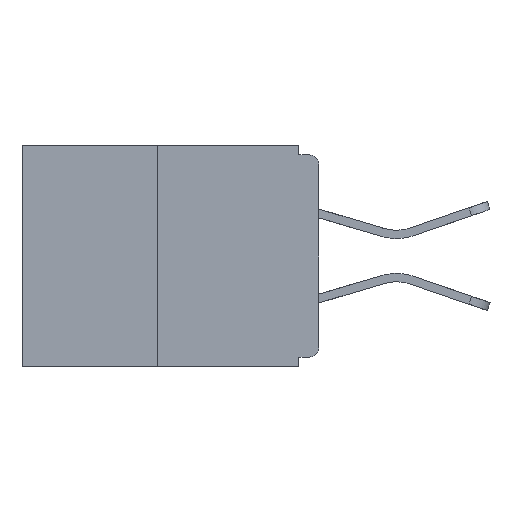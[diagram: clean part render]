
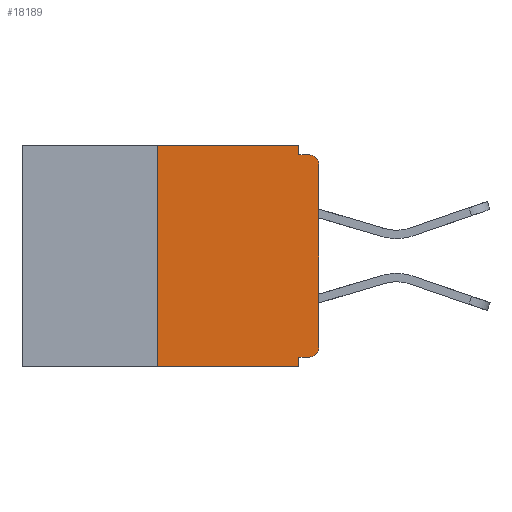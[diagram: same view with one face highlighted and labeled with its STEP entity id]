
A CAD part, left-side view. The second image highlights one B-rep face of the part: STEP entity #18189.
In plain terms, the highlighted planar face has unit normal (-1, 0, 0).
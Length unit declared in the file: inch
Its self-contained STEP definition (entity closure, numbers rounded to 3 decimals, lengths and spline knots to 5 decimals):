
#52 = VERTEX_POINT ( 'NONE', #10032 ) ;
#620 = CARTESIAN_POINT ( 'NONE',  ( 0., 0.015, -0.03 ) ) ;
#627 = DIRECTION ( 'NONE',  ( 0., 1., 0. ) ) ;
#785 = DIRECTION ( 'NONE',  ( 0., -1., 0. ) ) ;
#1181 = VECTOR ( 'NONE', #5397, 39.37008 ) ;
#1182 = AXIS2_PLACEMENT_3D ( 'NONE', #11232, #16362, #14877 ) ;
#1285 = CARTESIAN_POINT ( 'NONE',  ( 0., 0.015, -0.313 ) ) ;
#1603 = VECTOR ( 'NONE', #8721, 39.37008 ) ;
#1796 = EDGE_CURVE ( 'NONE', #11102, #2314, #11793, .T. ) ;
#2314 = VERTEX_POINT ( 'NONE', #2951 ) ;
#2432 = LINE ( 'NONE', #12105, #1603 ) ;
#2464 = PLANE ( 'NONE',  #1182 ) ;
#2807 = CARTESIAN_POINT ( 'NONE',  ( 0., 0.25, 0. ) ) ;
#2951 = CARTESIAN_POINT ( 'NONE',  ( 0., 0.031, -0.343 ) ) ;
#3135 = ORIENTED_EDGE ( 'NONE', *, *, #6657, .T. ) ;
#3842 = DIRECTION ( 'NONE',  ( 0., 0., 1. ) ) ;
#4138 = CARTESIAN_POINT ( 'NONE',  ( 0., 0.031, -0.343 ) ) ;
#4311 = EDGE_LOOP ( 'NONE', ( #10356, #5487, #3135, #16318, #19815, #11335, #14753, #18255, #19590, #19221 ) ) ;
#4668 = EDGE_CURVE ( 'NONE', #52, #5228, #10355, .T. ) ;
#4966 = FACE_OUTER_BOUND ( 'NONE', #4311, .T. ) ;
#5228 = VERTEX_POINT ( 'NONE', #5696 ) ;
#5397 = DIRECTION ( 'NONE',  ( 0., -1., 0. ) ) ;
#5487 = ORIENTED_EDGE ( 'NONE', *, *, #22257, .F. ) ;
#5653 = DIRECTION ( 'NONE',  ( 0., 0., -1. ) ) ;
#5679 = CARTESIAN_POINT ( 'NONE',  ( 0., 0., -0.313 ) ) ;
#5696 = CARTESIAN_POINT ( 'NONE',  ( 0., 0.015, -0.015 ) ) ;
#6507 = AXIS2_PLACEMENT_3D ( 'NONE', #1285, #7897, #7832 ) ;
#6517 = LINE ( 'NONE', #17927, #19963 ) ;
#6657 = EDGE_CURVE ( 'NONE', #22185, #2314, #14113, .T. ) ;
#6811 = LINE ( 'NONE', #17687, #15158 ) ;
#7174 = AXIS2_PLACEMENT_3D ( 'NONE', #620, #7460, #5653 ) ;
#7367 = DIRECTION ( 'NONE',  ( 0., 0., -1. ) ) ;
#7460 = DIRECTION ( 'NONE',  ( -1., 0., 0. ) ) ;
#7615 = VERTEX_POINT ( 'NONE', #15777 ) ;
#7832 = DIRECTION ( 'NONE',  ( 0., 0., -1. ) ) ;
#7897 = DIRECTION ( 'NONE',  ( -1., 0., 0. ) ) ;
#8721 = DIRECTION ( 'NONE',  ( 0., -1., 0. ) ) ;
#8995 = VERTEX_POINT ( 'NONE', #2807 ) ;
#9197 = CARTESIAN_POINT ( 'NONE',  ( 0., 0.25, 0. ) ) ;
#9594 = EDGE_CURVE ( 'NONE', #12391, #11303, #10916, .T. ) ;
#10032 = CARTESIAN_POINT ( 'NONE',  ( 0., 0., -0.03 ) ) ;
#10355 = CIRCLE ( 'NONE', #7174, 0.015 ) ;
#10356 = ORIENTED_EDGE ( 'NONE', *, *, #20700, .F. ) ;
#10426 = CARTESIAN_POINT ( 'NONE',  ( 0., 0.46, -0.343 ) ) ;
#10916 = CIRCLE ( 'NONE', #6507, 0.015 ) ;
#11055 = CARTESIAN_POINT ( 'NONE',  ( 0., 0., -0.328 ) ) ;
#11102 = VERTEX_POINT ( 'NONE', #11344 ) ;
#11232 = CARTESIAN_POINT ( 'NONE',  ( 0., 0.46, 0. ) ) ;
#11303 = VERTEX_POINT ( 'NONE', #5679 ) ;
#11335 = ORIENTED_EDGE ( 'NONE', *, *, #9594, .T. ) ;
#11344 = CARTESIAN_POINT ( 'NONE',  ( 0., 0.031, -0.328 ) ) ;
#11608 = EDGE_CURVE ( 'NONE', #11303, #52, #18665, .T. ) ;
#11726 = DIRECTION ( 'NONE',  ( 0., 0., 1. ) ) ;
#11793 = LINE ( 'NONE', #4138, #21533 ) ;
#12105 = CARTESIAN_POINT ( 'NONE',  ( 0., 0., -0.015 ) ) ;
#12391 = VERTEX_POINT ( 'NONE', #16953 ) ;
#14113 = LINE ( 'NONE', #10426, #1181 ) ;
#14308 = DIRECTION ( 'NONE',  ( 0., 0., -1. ) ) ;
#14350 = EDGE_CURVE ( 'NONE', #15071, #5228, #2432, .T. ) ;
#14753 = ORIENTED_EDGE ( 'NONE', *, *, #11608, .T. ) ;
#14877 = DIRECTION ( 'NONE',  ( 0., 0., -1. ) ) ;
#15071 = VERTEX_POINT ( 'NONE', #21362 ) ;
#15158 = VECTOR ( 'NONE', #7367, 39.37008 ) ;
#15777 = CARTESIAN_POINT ( 'NONE',  ( 0., 0.031, 0. ) ) ;
#16318 = ORIENTED_EDGE ( 'NONE', *, *, #1796, .F. ) ;
#16362 = DIRECTION ( 'NONE',  ( 1., 0., 0. ) ) ;
#16463 = VECTOR ( 'NONE', #627, 39.37008 ) ;
#16953 = CARTESIAN_POINT ( 'NONE',  ( 0., 0.015, -0.328 ) ) ;
#17687 = CARTESIAN_POINT ( 'NONE',  ( 0., 0.031, 0. ) ) ;
#17927 = CARTESIAN_POINT ( 'NONE',  ( 0., 0.46, 0. ) ) ;
#18105 = LINE ( 'NONE', #11055, #16463 ) ;
#18189 = ADVANCED_FACE ( 'NONE', ( #4966 ), #2464, .F. ) ;
#18255 = ORIENTED_EDGE ( 'NONE', *, *, #4668, .T. ) ;
#18665 = LINE ( 'NONE', #22080, #21650 ) ;
#19221 = ORIENTED_EDGE ( 'NONE', *, *, #19285, .F. ) ;
#19285 = EDGE_CURVE ( 'NONE', #7615, #15071, #6811, .T. ) ;
#19590 = ORIENTED_EDGE ( 'NONE', *, *, #14350, .F. ) ;
#19815 = ORIENTED_EDGE ( 'NONE', *, *, #20694, .F. ) ;
#19963 = VECTOR ( 'NONE', #785, 39.37008 ) ;
#20169 = LINE ( 'NONE', #9197, #20436 ) ;
#20436 = VECTOR ( 'NONE', #3842, 39.37008 ) ;
#20694 = EDGE_CURVE ( 'NONE', #12391, #11102, #18105, .T. ) ;
#20700 = EDGE_CURVE ( 'NONE', #8995, #7615, #6517, .T. ) ;
#20729 = CARTESIAN_POINT ( 'NONE',  ( 0., 0.25, -0.343 ) ) ;
#21362 = CARTESIAN_POINT ( 'NONE',  ( 0., 0.031, -0.015 ) ) ;
#21533 = VECTOR ( 'NONE', #14308, 39.37008 ) ;
#21650 = VECTOR ( 'NONE', #11726, 39.37008 ) ;
#22080 = CARTESIAN_POINT ( 'NONE',  ( 0., 0., 0. ) ) ;
#22185 = VERTEX_POINT ( 'NONE', #20729 ) ;
#22257 = EDGE_CURVE ( 'NONE', #22185, #8995, #20169, .T. ) ;
